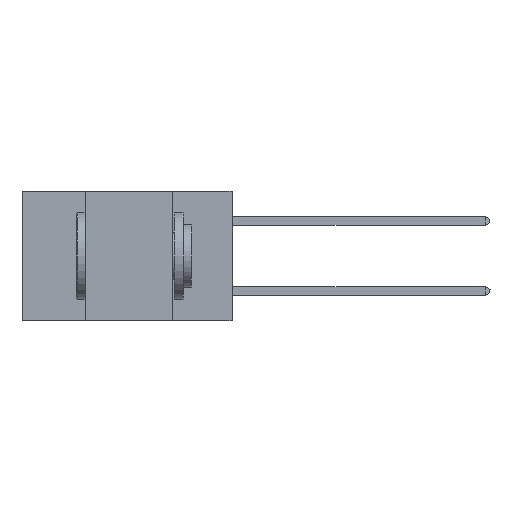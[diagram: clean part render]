
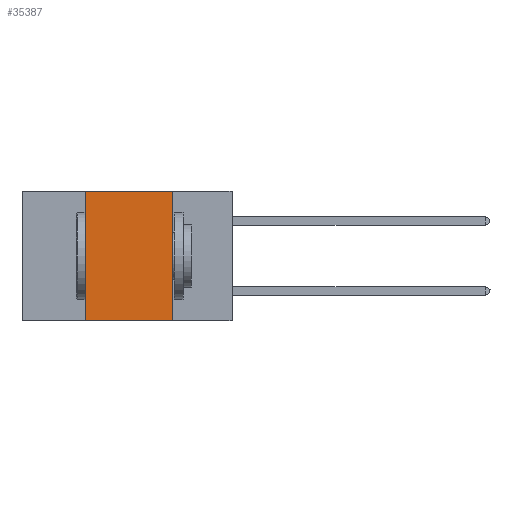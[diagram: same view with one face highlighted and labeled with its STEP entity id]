
A CAD part, left-side view. The second image highlights one B-rep face of the part: STEP entity #35387.
In plain terms, the highlighted planar face has unit normal (-1, 0, 0).
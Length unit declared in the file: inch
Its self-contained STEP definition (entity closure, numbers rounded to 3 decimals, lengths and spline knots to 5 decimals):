
#1377 = LINE ( 'NONE', #25148, #26953 ) ;
#1591 = AXIS2_PLACEMENT_3D ( 'NONE', #13200, #37136, #16727 ) ;
#2849 = VERTEX_POINT ( 'NONE', #6920 ) ;
#3803 = VECTOR ( 'NONE', #26938, 39.37008 ) ;
#5897 = CARTESIAN_POINT ( 'NONE',  ( 0., 0.17, 0. ) ) ;
#6454 = EDGE_CURVE ( 'NONE', #30341, #14841, #23236, .T. ) ;
#6920 = CARTESIAN_POINT ( 'NONE',  ( 0., 0.17, -0.37 ) ) ;
#13170 = LINE ( 'NONE', #43880, #3803 ) ;
#13200 = CARTESIAN_POINT ( 'NONE',  ( 0., 0.6, 0. ) ) ;
#14841 = VERTEX_POINT ( 'NONE', #30356 ) ;
#16727 = DIRECTION ( 'NONE',  ( 0., 0., -1. ) ) ;
#18432 = ORIENTED_EDGE ( 'NONE', *, *, #36745, .F. ) ;
#20212 = DIRECTION ( 'NONE',  ( 0., -1., 0. ) ) ;
#22240 = ORIENTED_EDGE ( 'NONE', *, *, #25258, .F. ) ;
#22900 = EDGE_CURVE ( 'NONE', #30341, #2849, #13170, .T. ) ;
#23236 = LINE ( 'NONE', #31914, #39183 ) ;
#25148 = CARTESIAN_POINT ( 'NONE',  ( 0., 0.17, 0. ) ) ;
#25258 = EDGE_CURVE ( 'NONE', #27568, #2849, #1377, .T. ) ;
#26752 = PLANE ( 'NONE',  #1591 ) ;
#26938 = DIRECTION ( 'NONE',  ( 0., -1., 0. ) ) ;
#26953 = VECTOR ( 'NONE', #38637, 39.37008 ) ;
#27568 = VERTEX_POINT ( 'NONE', #5897 ) ;
#30341 = VERTEX_POINT ( 'NONE', #42648 ) ;
#30356 = CARTESIAN_POINT ( 'NONE',  ( 0., 0.42, 0. ) ) ;
#31778 = ORIENTED_EDGE ( 'NONE', *, *, #6454, .F. ) ;
#31914 = CARTESIAN_POINT ( 'NONE',  ( 0., 0.42, 0. ) ) ;
#33331 = EDGE_LOOP ( 'NONE', ( #22240, #18432, #31778, #40802 ) ) ;
#35387 = ADVANCED_FACE ( 'NONE', ( #42329 ), #26752, .F. ) ;
#36745 = EDGE_CURVE ( 'NONE', #14841, #27568, #42204, .T. ) ;
#37136 = DIRECTION ( 'NONE',  ( 1., 0., 0. ) ) ;
#37175 = CARTESIAN_POINT ( 'NONE',  ( 0., 0.6, 0. ) ) ;
#38637 = DIRECTION ( 'NONE',  ( 0., 0., -1. ) ) ;
#38737 = DIRECTION ( 'NONE',  ( 0., 0., 1. ) ) ;
#38994 = VECTOR ( 'NONE', #20212, 39.37008 ) ;
#39183 = VECTOR ( 'NONE', #38737, 39.37008 ) ;
#40802 = ORIENTED_EDGE ( 'NONE', *, *, #22900, .T. ) ;
#42204 = LINE ( 'NONE', #37175, #38994 ) ;
#42329 = FACE_OUTER_BOUND ( 'NONE', #33331, .T. ) ;
#42648 = CARTESIAN_POINT ( 'NONE',  ( 0., 0.42, -0.37 ) ) ;
#43880 = CARTESIAN_POINT ( 'NONE',  ( 0., 0.6, -0.37 ) ) ;
